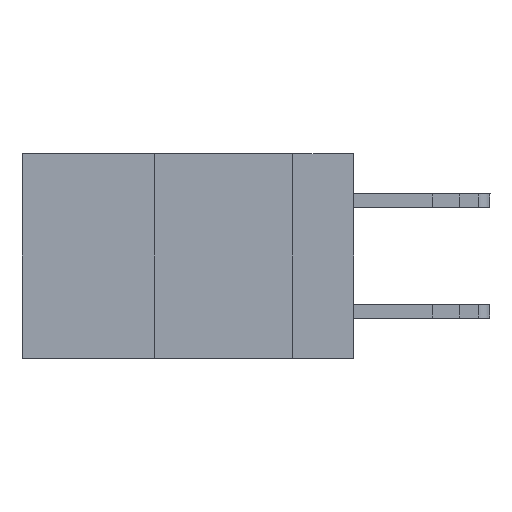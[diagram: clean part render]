
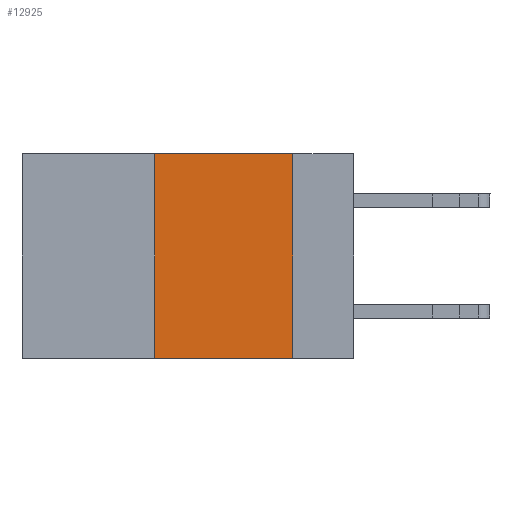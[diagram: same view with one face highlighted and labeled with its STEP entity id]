
A CAD part, left-side view. The second image highlights one B-rep face of the part: STEP entity #12925.
In plain terms, the highlighted planar face has unit normal (-1, 0, 0).
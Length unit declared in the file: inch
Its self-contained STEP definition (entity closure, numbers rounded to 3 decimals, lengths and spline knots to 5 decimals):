
#77 = VERTEX_POINT ( 'NONE', #19140 ) ;
#1227 = CARTESIAN_POINT ( 'NONE',  ( 0., 0.6, -0.37 ) ) ;
#1829 = DIRECTION ( 'NONE',  ( 0., 0., 1. ) ) ;
#2907 = VERTEX_POINT ( 'NONE', #3504 ) ;
#2944 = LINE ( 'NONE', #28114, #21741 ) ;
#3504 = CARTESIAN_POINT ( 'NONE',  ( 0., 0.36, 0. ) ) ;
#3949 = PLANE ( 'NONE',  #20694 ) ;
#3962 = EDGE_CURVE ( 'NONE', #2907, #30770, #19176, .T. ) ;
#4898 = ORIENTED_EDGE ( 'NONE', *, *, #5289, .T. ) ;
#5289 = EDGE_CURVE ( 'NONE', #22930, #77, #24297, .T. ) ;
#5579 = DIRECTION ( 'NONE',  ( 0., 0., -1. ) ) ;
#5590 = VECTOR ( 'NONE', #33559, 39.37008 ) ;
#6639 = LINE ( 'NONE', #29738, #12737 ) ;
#9442 = DIRECTION ( 'NONE',  ( 1., 0., 0. ) ) ;
#10092 = FACE_OUTER_BOUND ( 'NONE', #13779, .T. ) ;
#10175 = EDGE_CURVE ( 'NONE', #30770, #77, #2944, .T. ) ;
#12170 = EDGE_CURVE ( 'NONE', #22930, #2907, #6639, .T. ) ;
#12737 = VECTOR ( 'NONE', #1829, 39.37008 ) ;
#12882 = VECTOR ( 'NONE', #18471, 39.37008 ) ;
#12925 = ADVANCED_FACE ( 'NONE', ( #10092 ), #3949, .F. ) ;
#13779 = EDGE_LOOP ( 'NONE', ( #22754, #27612, #16030, #4898 ) ) ;
#15130 = CARTESIAN_POINT ( 'NONE',  ( 0., 0.6, 0. ) ) ;
#16030 = ORIENTED_EDGE ( 'NONE', *, *, #12170, .F. ) ;
#18471 = DIRECTION ( 'NONE',  ( 0., -1., 0. ) ) ;
#18501 = CARTESIAN_POINT ( 'NONE',  ( 0., 0.11, 0. ) ) ;
#19140 = CARTESIAN_POINT ( 'NONE',  ( 0., 0.11, -0.37 ) ) ;
#19176 = LINE ( 'NONE', #25178, #5590 ) ;
#20694 = AXIS2_PLACEMENT_3D ( 'NONE', #15130, #9442, #23760 ) ;
#20725 = CARTESIAN_POINT ( 'NONE',  ( 0., 0.36, -0.37 ) ) ;
#21741 = VECTOR ( 'NONE', #5579, 39.37008 ) ;
#22754 = ORIENTED_EDGE ( 'NONE', *, *, #10175, .F. ) ;
#22930 = VERTEX_POINT ( 'NONE', #20725 ) ;
#23760 = DIRECTION ( 'NONE',  ( 0., 0., -1. ) ) ;
#24297 = LINE ( 'NONE', #1227, #12882 ) ;
#25178 = CARTESIAN_POINT ( 'NONE',  ( 0., 0.6, 0. ) ) ;
#27612 = ORIENTED_EDGE ( 'NONE', *, *, #3962, .F. ) ;
#28114 = CARTESIAN_POINT ( 'NONE',  ( 0., 0.11, 0. ) ) ;
#29738 = CARTESIAN_POINT ( 'NONE',  ( 0., 0.36, 0. ) ) ;
#30770 = VERTEX_POINT ( 'NONE', #18501 ) ;
#33559 = DIRECTION ( 'NONE',  ( 0., -1., 0. ) ) ;
